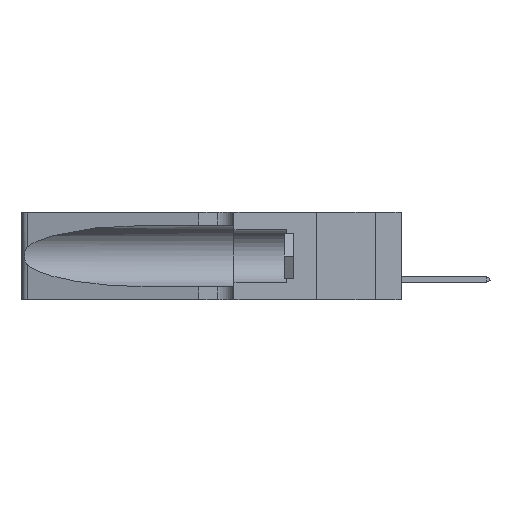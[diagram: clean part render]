
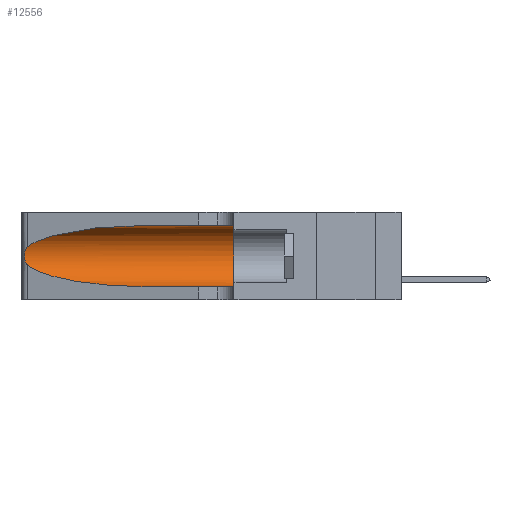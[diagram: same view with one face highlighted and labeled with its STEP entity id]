
A CAD part, left-side view. The second image highlights one B-rep face of the part: STEP entity #12556.
In plain terms, the highlighted cylindrical face has radius 3.308 mm (diameter 6.617 mm), a partial arc.
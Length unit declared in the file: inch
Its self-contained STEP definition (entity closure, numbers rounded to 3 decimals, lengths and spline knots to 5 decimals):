
#14 = CARTESIAN_POINT ( 'NONE',  ( 0.26018, 1.23835, 0.19895 ) ) ;
#85 = CARTESIAN_POINT ( 'NONE',  ( 0.25639, 1.23186, 0.15144 ) ) ;
#110 = CARTESIAN_POINT ( 'NONE',  ( 0.1305, 0.35, 0.31525 ) ) ;
#153 = CARTESIAN_POINT ( 'NONE',  ( 0.25639, 1.23184, 0.21858 ) ) ;
#681 = DIRECTION ( 'NONE',  ( 0., -1., 0. ) ) ;
#1012 = EDGE_CURVE ( 'NONE', #14681, #14885, #2918, .T. ) ;
#1995 = CARTESIAN_POINT ( 'NONE',  ( 0.25487, 1.22718, 0.22369 ) ) ;
#2216 = CARTESIAN_POINT ( 'NONE',  ( 0.25487, 1.22718, 0.22369 ) ) ;
#2461 = DIRECTION ( 'NONE',  ( 0., -1., 0. ) ) ;
#2918 = B_SPLINE_CURVE_WITH_KNOTS ( 'NONE', 3,
 ( #1995, #3818, #153, #18103, #21863, #14, #5468, #10996, #7298, #21717, #3742, #85, #12760, #21791 ),
 .UNSPECIFIED., .F., .F.,
 ( 4, 2, 2, 2, 2, 2, 4 ),
 ( 0., 0.00027, 0.00053, 0.00107, 0.0016, 0.00187, 0.00214 ),
 .UNSPECIFIED. ) ;
#3354 = FACE_OUTER_BOUND ( 'NONE', #19181, .T. ) ;
#3521 = ORIENTED_EDGE ( 'NONE', *, *, #23343, .T. ) ;
#3742 = CARTESIAN_POINT ( 'NONE',  ( 0.25789, 1.23486, 0.15765 ) ) ;
#3818 = CARTESIAN_POINT ( 'NONE',  ( 0.25555, 1.22994, 0.2215 ) ) ;
#4007 = ORIENTED_EDGE ( 'NONE', *, *, #22277, .F. ) ;
#4335 =( BOUNDED_CURVE ( )  B_SPLINE_CURVE ( 3, ( #22097, #13289, #6005, #20364 ),
 .UNSPECIFIED., .F., .F. ) 
 B_SPLINE_CURVE_WITH_KNOTS ( ( 4, 4 ),
 ( 3.44316, 4.71239 ),
 .UNSPECIFIED. ) 
 CURVE ( )  GEOMETRIC_REPRESENTATION_ITEM ( )  RATIONAL_B_SPLINE_CURVE ( ( 1., 0.87, 0.87, 1. ) ) 
 REPRESENTATION_ITEM ( '' )  );
#5380 = CARTESIAN_POINT ( 'NONE',  ( 0.1305, 0.72297, 0.31525 ) ) ;
#5468 = CARTESIAN_POINT ( 'NONE',  ( 0.26075, 1.23896, 0.19203 ) ) ;
#6005 = CARTESIAN_POINT ( 'NONE',  ( 0.18966, 0.96281, 0.05475 ) ) ;
#6064 = VERTEX_POINT ( 'NONE', #5380 ) ;
#7298 = CARTESIAN_POINT ( 'NONE',  ( 0.26017, 1.23833, 0.17102 ) ) ;
#8142 = ORIENTED_EDGE ( 'NONE', *, *, #13762, .T. ) ;
#8498 = CARTESIAN_POINT ( 'NONE',  ( 0.25487, 1.22718, 0.22369 ) ) ;
#9117 = CIRCLE ( 'NONE', #11017, 0.13025 ) ;
#10996 = CARTESIAN_POINT ( 'NONE',  ( 0.26075, 1.23896, 0.178 ) ) ;
#11017 = AXIS2_PLACEMENT_3D ( 'NONE', #11586, #18741, #11809 ) ;
#11139 = ORIENTED_EDGE ( 'NONE', *, *, #1012, .T. ) ;
#11446 = CARTESIAN_POINT ( 'NONE',  ( 0.1305, 1.61858, 0.05475 ) ) ;
#11586 = CARTESIAN_POINT ( 'NONE',  ( 0.1305, 0.35, 0.185 ) ) ;
#11809 = DIRECTION ( 'NONE',  ( 0., 0., 1. ) ) ;
#11901 = CARTESIAN_POINT ( 'NONE',  ( 0.25487, 1.22718, 0.14631 ) ) ;
#12010 =( BOUNDED_CURVE ( )  B_SPLINE_CURVE ( 3, ( #19455, #14334, #16132, #8498 ),
 .UNSPECIFIED., .F., .F. ) 
 B_SPLINE_CURVE_WITH_KNOTS ( ( 4, 4 ),
 ( 1.5708, 2.84003 ),
 .UNSPECIFIED. ) 
 CURVE ( )  GEOMETRIC_REPRESENTATION_ITEM ( )  RATIONAL_B_SPLINE_CURVE ( ( 1., 0.87, 0.87, 1. ) ) 
 REPRESENTATION_ITEM ( '' )  );
#12556 = ADVANCED_FACE ( 'NONE', ( #3354 ), #18810, .F. ) ;
#12760 = CARTESIAN_POINT ( 'NONE',  ( 0.25555, 1.22993, 0.14849 ) ) ;
#12922 = ORIENTED_EDGE ( 'NONE', *, *, #23350, .T. ) ;
#13272 = CARTESIAN_POINT ( 'NONE',  ( 0.1305, 0.35, 0.05475 ) ) ;
#13289 = CARTESIAN_POINT ( 'NONE',  ( 0.2373, 1.15595, 0.08982 ) ) ;
#13300 = CARTESIAN_POINT ( 'NONE',  ( 0.1305, 1.61858, 0.31525 ) ) ;
#13701 = LINE ( 'NONE', #13300, #14532 ) ;
#13762 = EDGE_CURVE ( 'NONE', #6064, #14681, #12010, .T. ) ;
#14334 = CARTESIAN_POINT ( 'NONE',  ( 0.18966, 0.96281, 0.31525 ) ) ;
#14532 = VECTOR ( 'NONE', #2461, 39.37008 ) ;
#14681 = VERTEX_POINT ( 'NONE', #2216 ) ;
#14885 = VERTEX_POINT ( 'NONE', #11901 ) ;
#15002 = DIRECTION ( 'NONE',  ( 0., -1., 0. ) ) ;
#15239 = AXIS2_PLACEMENT_3D ( 'NONE', #16789, #681, #18749 ) ;
#16087 = VERTEX_POINT ( 'NONE', #110 ) ;
#16132 = CARTESIAN_POINT ( 'NONE',  ( 0.2373, 1.15595, 0.28018 ) ) ;
#16646 = CARTESIAN_POINT ( 'NONE',  ( 0.1305, 0.72297, 0.05475 ) ) ;
#16789 = CARTESIAN_POINT ( 'NONE',  ( 0.1305, 1.61858, 0.185 ) ) ;
#17170 = ORIENTED_EDGE ( 'NONE', *, *, #20578, .F. ) ;
#17788 = VECTOR ( 'NONE', #15002, 39.37008 ) ;
#18103 = CARTESIAN_POINT ( 'NONE',  ( 0.25787, 1.23484, 0.2124 ) ) ;
#18741 = DIRECTION ( 'NONE',  ( 0., 1., 0. ) ) ;
#18749 = DIRECTION ( 'NONE',  ( 0., 0., -1. ) ) ;
#18810 = CYLINDRICAL_SURFACE ( 'NONE', #15239, 0.13025 ) ;
#19181 = EDGE_LOOP ( 'NONE', ( #8142, #11139, #12922, #3521, #4007, #17170 ) ) ;
#19204 = LINE ( 'NONE', #11446, #17788 ) ;
#19455 = CARTESIAN_POINT ( 'NONE',  ( 0.1305, 0.72297, 0.31525 ) ) ;
#20364 = CARTESIAN_POINT ( 'NONE',  ( 0.1305, 0.72297, 0.05475 ) ) ;
#20578 = EDGE_CURVE ( 'NONE', #6064, #16087, #13701, .T. ) ;
#21188 = VERTEX_POINT ( 'NONE', #13272 ) ;
#21200 = VERTEX_POINT ( 'NONE', #16646 ) ;
#21717 = CARTESIAN_POINT ( 'NONE',  ( 0.25856, 1.23593, 0.16098 ) ) ;
#21791 = CARTESIAN_POINT ( 'NONE',  ( 0.25487, 1.22718, 0.14631 ) ) ;
#21863 = CARTESIAN_POINT ( 'NONE',  ( 0.25854, 1.2359, 0.20912 ) ) ;
#22097 = CARTESIAN_POINT ( 'NONE',  ( 0.25487, 1.22718, 0.14631 ) ) ;
#22277 = EDGE_CURVE ( 'NONE', #16087, #21188, #9117, .T. ) ;
#23343 = EDGE_CURVE ( 'NONE', #21200, #21188, #19204, .T. ) ;
#23350 = EDGE_CURVE ( 'NONE', #14885, #21200, #4335, .T. ) ;
